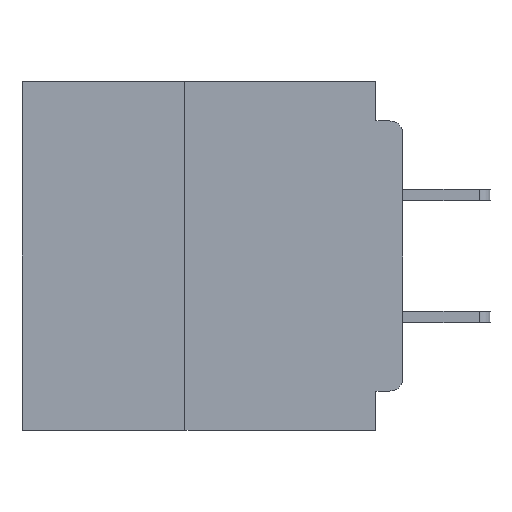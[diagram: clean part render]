
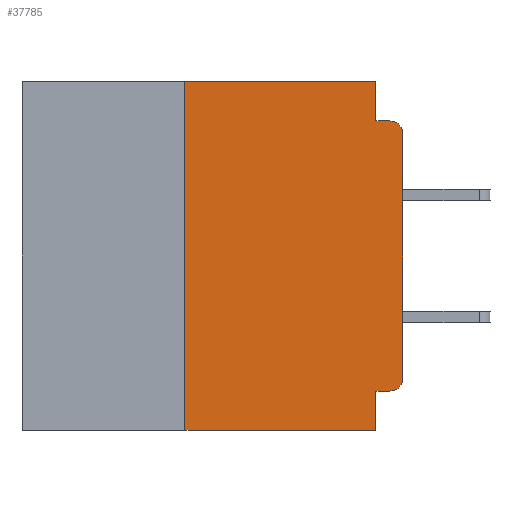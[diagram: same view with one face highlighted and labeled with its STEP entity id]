
A CAD part, left-side view. The second image highlights one B-rep face of the part: STEP entity #37785.
In plain terms, the highlighted planar face has unit normal (-1, 0, 0).
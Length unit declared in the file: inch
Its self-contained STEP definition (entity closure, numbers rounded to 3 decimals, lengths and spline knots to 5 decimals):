
#224 = ORIENTED_EDGE ( 'NONE', *, *, #7358, .F. ) ;
#356 = EDGE_CURVE ( 'NONE', #23093, #41295, #30628, .T. ) ;
#920 = CARTESIAN_POINT ( 'NONE',  ( 0., 0., -0.34 ) ) ;
#1224 = CARTESIAN_POINT ( 'NONE',  ( 0., 0.437, 0. ) ) ;
#2409 = VERTEX_POINT ( 'NONE', #41354 ) ;
#3970 = DIRECTION ( 'NONE',  ( 0., -1., 0. ) ) ;
#5297 = ORIENTED_EDGE ( 'NONE', *, *, #58827, .F. ) ;
#5624 = VECTOR ( 'NONE', #9752, 39.37008 ) ;
#5814 = VECTOR ( 'NONE', #3970, 39.37008 ) ;
#5845 = EDGE_CURVE ( 'NONE', #41568, #15655, #42540, .T. ) ;
#6389 = DIRECTION ( 'NONE',  ( 0., 0., -1. ) ) ;
#6657 = DIRECTION ( 'NONE',  ( 0., 0., -1. ) ) ;
#6966 = EDGE_CURVE ( 'NONE', #23093, #27550, #34448, .T. ) ;
#7358 = EDGE_CURVE ( 'NONE', #41295, #49687, #52806, .T. ) ;
#7876 = ORIENTED_EDGE ( 'NONE', *, *, #31620, .F. ) ;
#9567 = CARTESIAN_POINT ( 'NONE',  ( 0., 0.015, -0.045 ) ) ;
#9752 = DIRECTION ( 'NONE',  ( 0., 1., 0. ) ) ;
#9788 = LINE ( 'NONE', #36617, #58326 ) ;
#10450 = LINE ( 'NONE', #35968, #59014 ) ;
#10735 = DIRECTION ( 'NONE',  ( 0., 0., -1. ) ) ;
#13135 = DIRECTION ( 'NONE',  ( -1., 0., 0. ) ) ;
#15655 = VERTEX_POINT ( 'NONE', #17298 ) ;
#15750 = CARTESIAN_POINT ( 'NONE',  ( 0., 0.25, 0. ) ) ;
#17298 = CARTESIAN_POINT ( 'NONE',  ( 0., 0.031, 0. ) ) ;
#22624 = DIRECTION ( 'NONE',  ( 0., -1., 0. ) ) ;
#22637 = CARTESIAN_POINT ( 'NONE',  ( 0., 0.437, -0.4 ) ) ;
#23093 = VERTEX_POINT ( 'NONE', #38385 ) ;
#23119 = DIRECTION ( 'NONE',  ( -1., 0., 0. ) ) ;
#23581 = CARTESIAN_POINT ( 'NONE',  ( 0., 0., -0.355 ) ) ;
#25072 = PLANE ( 'NONE',  #50754 ) ;
#26849 = LINE ( 'NONE', #51395, #59955 ) ;
#27550 = VERTEX_POINT ( 'NONE', #920 ) ;
#28589 = VECTOR ( 'NONE', #38786, 39.37008 ) ;
#29465 = CARTESIAN_POINT ( 'NONE',  ( 0., 0.031, 0. ) ) ;
#29834 = CARTESIAN_POINT ( 'NONE',  ( 0., 0.437, 0. ) ) ;
#29896 = ORIENTED_EDGE ( 'NONE', *, *, #5845, .F. ) ;
#30628 = LINE ( 'NONE', #23581, #5624 ) ;
#31620 = EDGE_CURVE ( 'NONE', #15655, #2409, #59459, .T. ) ;
#33136 = ORIENTED_EDGE ( 'NONE', *, *, #6966, .T. ) ;
#34019 = VERTEX_POINT ( 'NONE', #9567 ) ;
#34397 = VECTOR ( 'NONE', #10735, 39.37008 ) ;
#34448 = CIRCLE ( 'NONE', #55836, 0.015 ) ;
#34503 = DIRECTION ( 'NONE',  ( 1., 0., 0. ) ) ;
#34950 = EDGE_CURVE ( 'NONE', #46572, #41568, #10450, .T. ) ;
#35869 = VECTOR ( 'NONE', #6657, 39.37008 ) ;
#35968 = CARTESIAN_POINT ( 'NONE',  ( 0., 0.25, -0.4 ) ) ;
#36182 = DIRECTION ( 'NONE',  ( 0., 0., 1. ) ) ;
#36617 = CARTESIAN_POINT ( 'NONE',  ( 0., 0., -0.045 ) ) ;
#37470 = EDGE_CURVE ( 'NONE', #46572, #49687, #55831, .T. ) ;
#37785 = ADVANCED_FACE ( 'NONE', ( #38113 ), #25072, .F. ) ;
#38113 = FACE_OUTER_BOUND ( 'NONE', #55040, .T. ) ;
#38385 = CARTESIAN_POINT ( 'NONE',  ( 0., 0.015, -0.355 ) ) ;
#38582 = CIRCLE ( 'NONE', #45948, 0.015 ) ;
#38786 = DIRECTION ( 'NONE',  ( 0., -1., 0. ) ) ;
#40578 = CARTESIAN_POINT ( 'NONE',  ( 0., 0., -0.06 ) ) ;
#41275 = CARTESIAN_POINT ( 'NONE',  ( 0., 0.015, -0.06 ) ) ;
#41295 = VERTEX_POINT ( 'NONE', #42104 ) ;
#41354 = CARTESIAN_POINT ( 'NONE',  ( 0., 0.031, -0.045 ) ) ;
#41568 = VERTEX_POINT ( 'NONE', #15750 ) ;
#42104 = CARTESIAN_POINT ( 'NONE',  ( 0., 0.031, -0.355 ) ) ;
#42540 = LINE ( 'NONE', #1224, #28589 ) ;
#45093 = ORIENTED_EDGE ( 'NONE', *, *, #356, .F. ) ;
#45613 = EDGE_CURVE ( 'NONE', #27550, #59931, #26849, .T. ) ;
#45948 = AXIS2_PLACEMENT_3D ( 'NONE', #41275, #13135, #46018 ) ;
#46018 = DIRECTION ( 'NONE',  ( 0., 0., -1. ) ) ;
#46572 = VERTEX_POINT ( 'NONE', #59128 ) ;
#46758 = ORIENTED_EDGE ( 'NONE', *, *, #34950, .F. ) ;
#47138 = ORIENTED_EDGE ( 'NONE', *, *, #37470, .T. ) ;
#47547 = ORIENTED_EDGE ( 'NONE', *, *, #45613, .T. ) ;
#49687 = VERTEX_POINT ( 'NONE', #58192 ) ;
#50754 = AXIS2_PLACEMENT_3D ( 'NONE', #29834, #34503, #6389 ) ;
#51305 = CARTESIAN_POINT ( 'NONE',  ( 0., 0.015, -0.34 ) ) ;
#51395 = CARTESIAN_POINT ( 'NONE',  ( 0., 0., 0. ) ) ;
#52806 = LINE ( 'NONE', #58650, #35869 ) ;
#55040 = EDGE_LOOP ( 'NONE', ( #47547, #60612, #5297, #7876, #29896, #46758, #47138, #224, #45093, #33136 ) ) ;
#55831 = LINE ( 'NONE', #22637, #5814 ) ;
#55836 = AXIS2_PLACEMENT_3D ( 'NONE', #51305, #23119, #56025 ) ;
#56025 = DIRECTION ( 'NONE',  ( 0., 0., -1. ) ) ;
#56334 = DIRECTION ( 'NONE',  ( 0., 0., 1. ) ) ;
#57035 = EDGE_CURVE ( 'NONE', #59931, #34019, #38582, .T. ) ;
#58192 = CARTESIAN_POINT ( 'NONE',  ( 0., 0.031, -0.4 ) ) ;
#58326 = VECTOR ( 'NONE', #22624, 39.37008 ) ;
#58650 = CARTESIAN_POINT ( 'NONE',  ( 0., 0.031, -0.4 ) ) ;
#58827 = EDGE_CURVE ( 'NONE', #2409, #34019, #9788, .T. ) ;
#59014 = VECTOR ( 'NONE', #36182, 39.37008 ) ;
#59128 = CARTESIAN_POINT ( 'NONE',  ( 0., 0.25, -0.4 ) ) ;
#59459 = LINE ( 'NONE', #29465, #34397 ) ;
#59931 = VERTEX_POINT ( 'NONE', #40578 ) ;
#59955 = VECTOR ( 'NONE', #56334, 39.37008 ) ;
#60612 = ORIENTED_EDGE ( 'NONE', *, *, #57035, .T. ) ;
